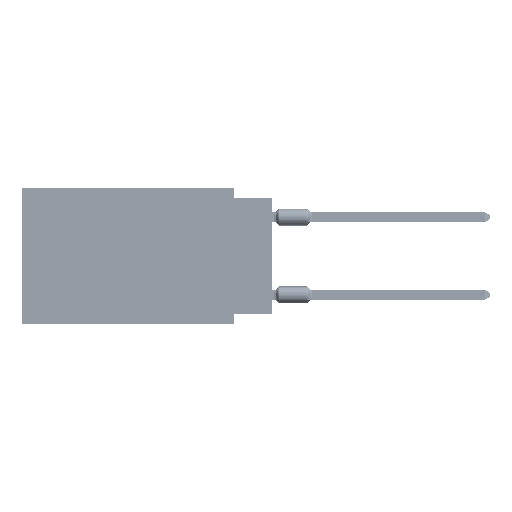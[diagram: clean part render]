
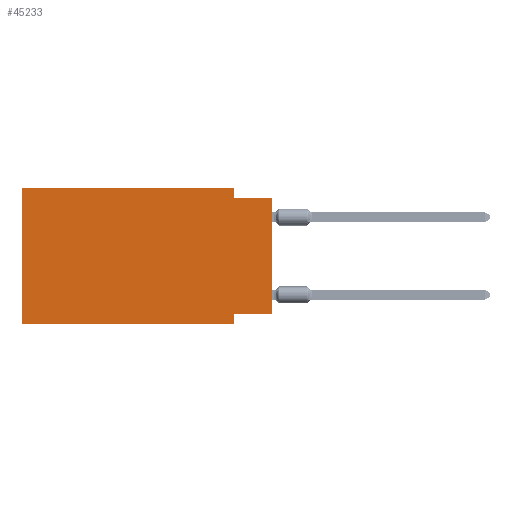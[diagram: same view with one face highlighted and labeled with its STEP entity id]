
A CAD part, left-side view. The second image highlights one B-rep face of the part: STEP entity #45233.
In plain terms, the highlighted planar face has unit normal (-1, 0, 0).
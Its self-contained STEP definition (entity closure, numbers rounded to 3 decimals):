
#225 = ORIENTED_EDGE ( 'NONE', *, *, #32741, .F. ) ;
#1137 = CARTESIAN_POINT ( 'NONE',  ( 0., 0., -8.255 ) ) ;
#4984 = VERTEX_POINT ( 'NONE', #36403 ) ;
#5029 = CARTESIAN_POINT ( 'NONE',  ( 0., 0., -0.635 ) ) ;
#7534 = PLANE ( 'NONE',  #46196 ) ;
#7651 = DIRECTION ( 'NONE',  ( 0., 0., 1. ) ) ;
#9311 = LINE ( 'NONE', #1137, #97631 ) ;
#10522 = VECTOR ( 'NONE', #78000, 1000. ) ;
#13324 = LINE ( 'NONE', #97852, #37494 ) ;
#15850 = EDGE_CURVE ( 'NONE', #76574, #68362, #81709, .T. ) ;
#19296 = VERTEX_POINT ( 'NONE', #103413 ) ;
#19548 = ORIENTED_EDGE ( 'NONE', *, *, #92144, .F. ) ;
#20542 = EDGE_LOOP ( 'NONE', ( #95362, #88870, #101254, #19548, #65590, #39123, #225, #25590 ) ) ;
#23338 = DIRECTION ( 'NONE',  ( 0., -1., 0. ) ) ;
#25357 = CARTESIAN_POINT ( 'NONE',  ( 0., 16.383, 0. ) ) ;
#25590 = ORIENTED_EDGE ( 'NONE', *, *, #51523, .F. ) ;
#26152 = CARTESIAN_POINT ( 'NONE',  ( 0., 2.54, 0. ) ) ;
#26724 = VECTOR ( 'NONE', #75243, 1000. ) ;
#32741 = EDGE_CURVE ( 'NONE', #54945, #68362, #13324, .T. ) ;
#34365 = EDGE_CURVE ( 'NONE', #19296, #4984, #79781, .T. ) ;
#34414 = DIRECTION ( 'NONE',  ( 0., 1., 0. ) ) ;
#34469 = CARTESIAN_POINT ( 'NONE',  ( 0., 2.54, 0. ) ) ;
#36403 = CARTESIAN_POINT ( 'NONE',  ( 0., 0., -0.635 ) ) ;
#37494 = VECTOR ( 'NONE', #63540, 1000. ) ;
#38320 = VERTEX_POINT ( 'NONE', #47402 ) ;
#39123 = ORIENTED_EDGE ( 'NONE', *, *, #15850, .T. ) ;
#40823 = VECTOR ( 'NONE', #55270, 1000. ) ;
#42187 = CARTESIAN_POINT ( 'NONE',  ( 0., 16.383, -8.89 ) ) ;
#45233 = ADVANCED_FACE ( 'NONE', ( #82297 ), #7534, .F. ) ;
#46196 = AXIS2_PLACEMENT_3D ( 'NONE', #107365, #90490, #65386 ) ;
#47402 = CARTESIAN_POINT ( 'NONE',  ( 0., 0., -8.255 ) ) ;
#48410 = CARTESIAN_POINT ( 'NONE',  ( 0., 16.383, -8.89 ) ) ;
#51523 = EDGE_CURVE ( 'NONE', #38320, #54945, #9311, .T. ) ;
#53452 = VECTOR ( 'NONE', #80872, 1000. ) ;
#54945 = VERTEX_POINT ( 'NONE', #84871 ) ;
#55270 = DIRECTION ( 'NONE',  ( 0., -1., 0. ) ) ;
#57587 = VERTEX_POINT ( 'NONE', #25357 ) ;
#58371 = EDGE_CURVE ( 'NONE', #76574, #57587, #82409, .T. ) ;
#63482 = LINE ( 'NONE', #70026, #40823 ) ;
#63540 = DIRECTION ( 'NONE',  ( 0., 0., -1. ) ) ;
#65386 = DIRECTION ( 'NONE',  ( 0., 0., -1. ) ) ;
#65590 = ORIENTED_EDGE ( 'NONE', *, *, #58371, .F. ) ;
#67991 = EDGE_CURVE ( 'NONE', #87107, #19296, #100858, .T. ) ;
#68362 = VERTEX_POINT ( 'NONE', #88815 ) ;
#70026 = CARTESIAN_POINT ( 'NONE',  ( 0., 16.383, 0. ) ) ;
#70381 = VECTOR ( 'NONE', #23338, 1000. ) ;
#75243 = DIRECTION ( 'NONE',  ( 0., 0., -1. ) ) ;
#76574 = VERTEX_POINT ( 'NONE', #42187 ) ;
#78000 = DIRECTION ( 'NONE',  ( 0., 0., 1. ) ) ;
#79781 = LINE ( 'NONE', #5029, #53452 ) ;
#80872 = DIRECTION ( 'NONE',  ( 0., -1., 0. ) ) ;
#81131 = EDGE_CURVE ( 'NONE', #38320, #4984, #85664, .T. ) ;
#81336 = CARTESIAN_POINT ( 'NONE',  ( 0., 16.383, 0. ) ) ;
#81709 = LINE ( 'NONE', #48410, #70381 ) ;
#82297 = FACE_OUTER_BOUND ( 'NONE', #20542, .T. ) ;
#82409 = LINE ( 'NONE', #81336, #92782 ) ;
#84871 = CARTESIAN_POINT ( 'NONE',  ( 0., 2.54, -8.255 ) ) ;
#85664 = LINE ( 'NONE', #93838, #10522 ) ;
#87107 = VERTEX_POINT ( 'NONE', #34469 ) ;
#88815 = CARTESIAN_POINT ( 'NONE',  ( 0., 2.54, -8.89 ) ) ;
#88870 = ORIENTED_EDGE ( 'NONE', *, *, #34365, .F. ) ;
#90490 = DIRECTION ( 'NONE',  ( 1., 0., 0. ) ) ;
#92144 = EDGE_CURVE ( 'NONE', #57587, #87107, #63482, .T. ) ;
#92782 = VECTOR ( 'NONE', #7651, 1000. ) ;
#93838 = CARTESIAN_POINT ( 'NONE',  ( 0., 0., 0. ) ) ;
#95362 = ORIENTED_EDGE ( 'NONE', *, *, #81131, .T. ) ;
#97631 = VECTOR ( 'NONE', #34414, 1000. ) ;
#97852 = CARTESIAN_POINT ( 'NONE',  ( 0., 2.54, -8.89 ) ) ;
#100858 = LINE ( 'NONE', #26152, #26724 ) ;
#101254 = ORIENTED_EDGE ( 'NONE', *, *, #67991, .F. ) ;
#103413 = CARTESIAN_POINT ( 'NONE',  ( 0., 2.54, -0.635 ) ) ;
#107365 = CARTESIAN_POINT ( 'NONE',  ( 0., 16.383, 0. ) ) ;
